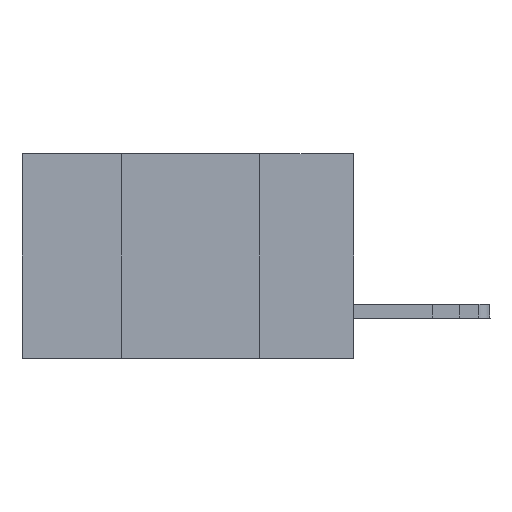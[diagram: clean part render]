
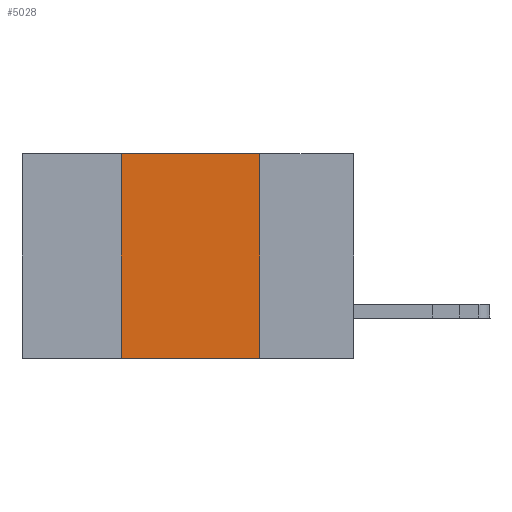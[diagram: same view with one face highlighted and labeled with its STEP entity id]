
A CAD part, left-side view. The second image highlights one B-rep face of the part: STEP entity #5028.
In plain terms, the highlighted planar face has unit normal (-1, 0, 0).
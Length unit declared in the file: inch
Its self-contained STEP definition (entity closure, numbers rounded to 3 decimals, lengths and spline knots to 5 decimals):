
#294 = ORIENTED_EDGE ( 'NONE', *, *, #8246, .F. ) ;
#567 = VECTOR ( 'NONE', #24005, 39.37008 ) ;
#1894 = PLANE ( 'NONE',  #6383 ) ;
#3085 = EDGE_CURVE ( 'NONE', #6734, #29562, #14102, .T. ) ;
#3594 = FACE_OUTER_BOUND ( 'NONE', #7354, .T. ) ;
#4665 = ORIENTED_EDGE ( 'NONE', *, *, #3085, .F. ) ;
#5028 = ADVANCED_FACE ( 'NONE', ( #3594 ), #1894, .F. ) ;
#6141 = DIRECTION ( 'NONE',  ( 0., -1., 0. ) ) ;
#6383 = AXIS2_PLACEMENT_3D ( 'NONE', #15747, #22665, #8952 ) ;
#6734 = VERTEX_POINT ( 'NONE', #13028 ) ;
#7354 = EDGE_LOOP ( 'NONE', ( #16495, #294, #4665, #12194 ) ) ;
#7727 = EDGE_CURVE ( 'NONE', #6734, #20222, #24640, .T. ) ;
#8246 = EDGE_CURVE ( 'NONE', #29562, #23081, #22452, .T. ) ;
#8952 = DIRECTION ( 'NONE',  ( 0., 0., -1. ) ) ;
#10338 = CARTESIAN_POINT ( 'NONE',  ( 0., 0.42, 0. ) ) ;
#10689 = DIRECTION ( 'NONE',  ( 0., -1., 0. ) ) ;
#12194 = ORIENTED_EDGE ( 'NONE', *, *, #7727, .T. ) ;
#13028 = CARTESIAN_POINT ( 'NONE',  ( 0., 0.42, -0.37 ) ) ;
#13383 = VECTOR ( 'NONE', #16670, 39.37008 ) ;
#13548 = CARTESIAN_POINT ( 'NONE',  ( 0., 0.17, 0. ) ) ;
#14102 = LINE ( 'NONE', #28127, #13383 ) ;
#15627 = VECTOR ( 'NONE', #6141, 39.37008 ) ;
#15747 = CARTESIAN_POINT ( 'NONE',  ( 0., 0.6, 0. ) ) ;
#16495 = ORIENTED_EDGE ( 'NONE', *, *, #28285, .F. ) ;
#16670 = DIRECTION ( 'NONE',  ( 0., 0., 1. ) ) ;
#18209 = LINE ( 'NONE', #21716, #567 ) ;
#20222 = VERTEX_POINT ( 'NONE', #22196 ) ;
#21716 = CARTESIAN_POINT ( 'NONE',  ( 0., 0.17, 0. ) ) ;
#22196 = CARTESIAN_POINT ( 'NONE',  ( 0., 0.17, -0.37 ) ) ;
#22452 = LINE ( 'NONE', #29004, #15627 ) ;
#22665 = DIRECTION ( 'NONE',  ( 1., 0., 0. ) ) ;
#23081 = VERTEX_POINT ( 'NONE', #13548 ) ;
#23913 = VECTOR ( 'NONE', #10689, 39.37008 ) ;
#24005 = DIRECTION ( 'NONE',  ( 0., 0., -1. ) ) ;
#24640 = LINE ( 'NONE', #29025, #23913 ) ;
#28127 = CARTESIAN_POINT ( 'NONE',  ( 0., 0.42, 0. ) ) ;
#28285 = EDGE_CURVE ( 'NONE', #23081, #20222, #18209, .T. ) ;
#29004 = CARTESIAN_POINT ( 'NONE',  ( 0., 0.6, 0. ) ) ;
#29025 = CARTESIAN_POINT ( 'NONE',  ( 0., 0.6, -0.37 ) ) ;
#29562 = VERTEX_POINT ( 'NONE', #10338 ) ;
